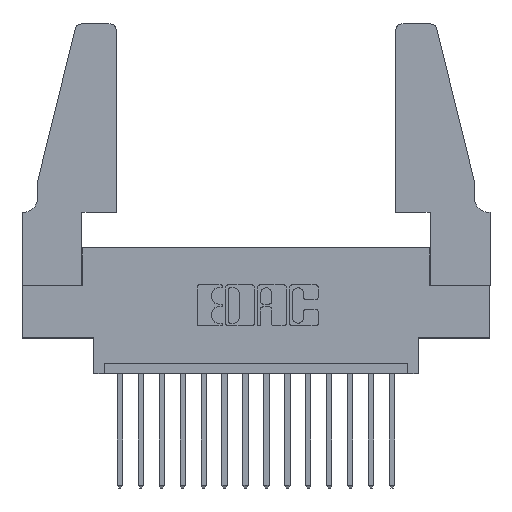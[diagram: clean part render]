
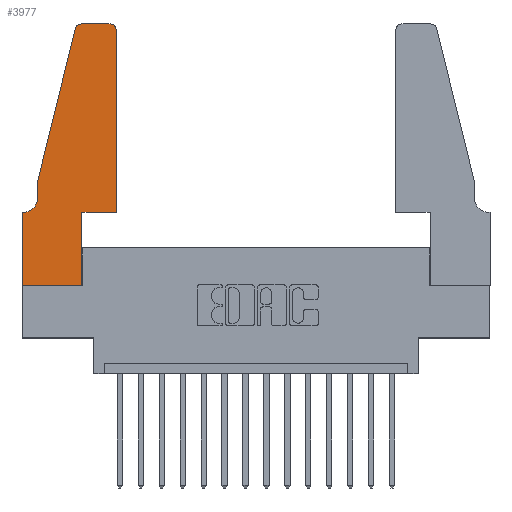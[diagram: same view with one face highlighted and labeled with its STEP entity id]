
A CAD part, top view. The second image highlights one B-rep face of the part: STEP entity #3977.
In plain terms, the highlighted planar face has unit normal (0, 0, 1).
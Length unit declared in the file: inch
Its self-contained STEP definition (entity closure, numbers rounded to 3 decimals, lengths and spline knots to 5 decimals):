
#444 = ORIENTED_EDGE ( 'NONE', *, *, #12407, .T. ) ;
#450 = CARTESIAN_POINT ( 'NONE',  ( 0.0755, 0.5, 0.37 ) ) ;
#571 = VERTEX_POINT ( 'NONE', #15454 ) ;
#788 = DIRECTION ( 'NONE',  ( -1., 0., 0. ) ) ;
#810 = VERTEX_POINT ( 'NONE', #12180 ) ;
#902 = CARTESIAN_POINT ( 'NONE',  ( 0.0755, 0.35, 0.37 ) ) ;
#979 = VERTEX_POINT ( 'NONE', #6836 ) ;
#1554 = CIRCLE ( 'NONE', #11083, 0.03 ) ;
#1864 = CARTESIAN_POINT ( 'NONE',  ( 0., 0., 0.37 ) ) ;
#2196 = LINE ( 'NONE', #10631, #14608 ) ;
#2213 = VECTOR ( 'NONE', #13676, 39.37008 ) ;
#2278 = CARTESIAN_POINT ( 'NONE',  ( 0.0055, 0.35, 0.37 ) ) ;
#2489 = DIRECTION ( 'NONE',  ( 0., 1., 0. ) ) ;
#3159 = CARTESIAN_POINT ( 'NONE',  ( 0.0755, 0.5, 0.37 ) ) ;
#3360 = EDGE_CURVE ( 'NONE', #9007, #979, #4590, .T. ) ;
#3392 = LINE ( 'NONE', #11049, #16000 ) ;
#3404 = EDGE_LOOP ( 'NONE', ( #8629, #16178, #14666, #444, #14325, #9494, #13981, #5302, #7642, #16197, #7687, #7142 ) ) ;
#3460 = CARTESIAN_POINT ( 'NONE',  ( 0.4505, 0.35, 0.37 ) ) ;
#3774 = AXIS2_PLACEMENT_3D ( 'NONE', #11562, #12553, #8917 ) ;
#3889 = CARTESIAN_POINT ( 'NONE',  ( 0.284, 1.25, 0.37 ) ) ;
#3894 = VERTEX_POINT ( 'NONE', #2278 ) ;
#3977 = ADVANCED_FACE ( 'NONE', ( #8327 ), #11458, .T. ) ;
#4134 = DIRECTION ( 'NONE',  ( 0., -1., 0. ) ) ;
#4146 = VECTOR ( 'NONE', #12476, 39.37008 ) ;
#4385 = CARTESIAN_POINT ( 'NONE',  ( 0.4205, 1.22, 0.37 ) ) ;
#4590 = CIRCLE ( 'NONE', #13576, 0.03 ) ;
#4602 = EDGE_CURVE ( 'NONE', #3894, #571, #8526, .T. ) ;
#4717 = CARTESIAN_POINT ( 'NONE',  ( 0.0755, 0.42, 0.37 ) ) ;
#4989 = CARTESIAN_POINT ( 'NONE',  ( 0.4505, 1.22, 0.37 ) ) ;
#5302 = ORIENTED_EDGE ( 'NONE', *, *, #15506, .T. ) ;
#5590 = LINE ( 'NONE', #1864, #2213 ) ;
#5667 = EDGE_CURVE ( 'NONE', #12551, #9007, #15120, .T. ) ;
#5698 = DIRECTION ( 'NONE',  ( 0., -1., 0. ) ) ;
#6191 = CIRCLE ( 'NONE', #9020, 0.07 ) ;
#6420 = VECTOR ( 'NONE', #11689, 39.37008 ) ;
#6467 = VECTOR ( 'NONE', #8378, 39.37008 ) ;
#6721 = VERTEX_POINT ( 'NONE', #4989 ) ;
#6766 = DIRECTION ( 'NONE',  ( 1., 0., 0. ) ) ;
#6836 = CARTESIAN_POINT ( 'NONE',  ( 0.25487, 1.22718, 0.37 ) ) ;
#7010 = VERTEX_POINT ( 'NONE', #12358 ) ;
#7142 = ORIENTED_EDGE ( 'NONE', *, *, #16295, .T. ) ;
#7149 = EDGE_CURVE ( 'NONE', #8238, #6721, #13042, .T. ) ;
#7272 = VECTOR ( 'NONE', #5698, 39.37008 ) ;
#7297 = DIRECTION ( 'NONE',  ( 1., 0., 0. ) ) ;
#7642 = ORIENTED_EDGE ( 'NONE', *, *, #7928, .T. ) ;
#7687 = ORIENTED_EDGE ( 'NONE', *, *, #7149, .T. ) ;
#7867 = LINE ( 'NONE', #3159, #6467 ) ;
#7928 = EDGE_CURVE ( 'NONE', #810, #9822, #14039, .T. ) ;
#8238 = VERTEX_POINT ( 'NONE', #3460 ) ;
#8327 = FACE_OUTER_BOUND ( 'NONE', #3404, .T. ) ;
#8378 = DIRECTION ( 'NONE',  ( -0.239, -0.971, 0. ) ) ;
#8393 = DIRECTION ( 'NONE',  ( 0., 0., -1. ) ) ;
#8526 = LINE ( 'NONE', #902, #4146 ) ;
#8551 = EDGE_CURVE ( 'NONE', #12487, #3894, #6191, .T. ) ;
#8629 = ORIENTED_EDGE ( 'NONE', *, *, #5667, .T. ) ;
#8897 = EDGE_CURVE ( 'NONE', #571, #12435, #2196, .T. ) ;
#8917 = DIRECTION ( 'NONE',  ( 1., 0., 0. ) ) ;
#9007 = VERTEX_POINT ( 'NONE', #3889 ) ;
#9020 = AXIS2_PLACEMENT_3D ( 'NONE', #15032, #8393, #12472 ) ;
#9494 = ORIENTED_EDGE ( 'NONE', *, *, #4602, .T. ) ;
#9822 = VERTEX_POINT ( 'NONE', #13778 ) ;
#10172 = CARTESIAN_POINT ( 'NONE',  ( 0.4505, 0.35, 0.37 ) ) ;
#10276 = EDGE_CURVE ( 'NONE', #9822, #8238, #3392, .T. ) ;
#10631 = CARTESIAN_POINT ( 'NONE',  ( 0., 0., 0.37 ) ) ;
#11049 = CARTESIAN_POINT ( 'NONE',  ( 0.4505, 0.35, 0.37 ) ) ;
#11083 = AXIS2_PLACEMENT_3D ( 'NONE', #4385, #13176, #6766 ) ;
#11458 = PLANE ( 'NONE',  #3774 ) ;
#11562 = CARTESIAN_POINT ( 'NONE',  ( 0., 0.35, 0.37 ) ) ;
#11689 = DIRECTION ( 'NONE',  ( 0., 1., 0. ) ) ;
#12035 = DIRECTION ( 'NONE',  ( 1., 0., 0. ) ) ;
#12180 = CARTESIAN_POINT ( 'NONE',  ( 0.2865, 0., 0.37 ) ) ;
#12242 = VECTOR ( 'NONE', #2489, 39.37008 ) ;
#12358 = CARTESIAN_POINT ( 'NONE',  ( 0.0755, 0.5, 0.37 ) ) ;
#12407 = EDGE_CURVE ( 'NONE', #7010, #12487, #15523, .T. ) ;
#12435 = VERTEX_POINT ( 'NONE', #15975 ) ;
#12470 = VECTOR ( 'NONE', #788, 39.37008 ) ;
#12472 = DIRECTION ( 'NONE',  ( -1., 0., 0. ) ) ;
#12476 = DIRECTION ( 'NONE',  ( -1., 0., 0. ) ) ;
#12487 = VERTEX_POINT ( 'NONE', #4717 ) ;
#12551 = VERTEX_POINT ( 'NONE', #15083 ) ;
#12553 = DIRECTION ( 'NONE',  ( 0., 0., 1. ) ) ;
#12904 = CARTESIAN_POINT ( 'NONE',  ( 0.2865, 0.35, 0.37 ) ) ;
#13042 = LINE ( 'NONE', #10172, #12242 ) ;
#13176 = DIRECTION ( 'NONE',  ( 0., 0., 1. ) ) ;
#13576 = AXIS2_PLACEMENT_3D ( 'NONE', #14892, #16112, #7297 ) ;
#13676 = DIRECTION ( 'NONE',  ( 1., 0., 0. ) ) ;
#13677 = EDGE_CURVE ( 'NONE', #979, #7010, #7867, .T. ) ;
#13778 = CARTESIAN_POINT ( 'NONE',  ( 0.2865, 0.35, 0.37 ) ) ;
#13981 = ORIENTED_EDGE ( 'NONE', *, *, #8897, .T. ) ;
#14039 = LINE ( 'NONE', #12904, #6420 ) ;
#14325 = ORIENTED_EDGE ( 'NONE', *, *, #8551, .T. ) ;
#14608 = VECTOR ( 'NONE', #4134, 39.37008 ) ;
#14666 = ORIENTED_EDGE ( 'NONE', *, *, #13677, .T. ) ;
#14892 = CARTESIAN_POINT ( 'NONE',  ( 0.284, 1.22, 0.37 ) ) ;
#15032 = CARTESIAN_POINT ( 'NONE',  ( 0.0055, 0.42, 0.37 ) ) ;
#15083 = CARTESIAN_POINT ( 'NONE',  ( 0.4205, 1.25, 0.37 ) ) ;
#15120 = LINE ( 'NONE', #15826, #12470 ) ;
#15454 = CARTESIAN_POINT ( 'NONE',  ( 0., 0.35, 0.37 ) ) ;
#15506 = EDGE_CURVE ( 'NONE', #12435, #810, #5590, .T. ) ;
#15523 = LINE ( 'NONE', #450, #7272 ) ;
#15826 = CARTESIAN_POINT ( 'NONE',  ( 0.2605, 1.25, 0.37 ) ) ;
#15975 = CARTESIAN_POINT ( 'NONE',  ( 0., 0., 0.37 ) ) ;
#16000 = VECTOR ( 'NONE', #12035, 39.37008 ) ;
#16112 = DIRECTION ( 'NONE',  ( 0., 0., 1. ) ) ;
#16178 = ORIENTED_EDGE ( 'NONE', *, *, #3360, .T. ) ;
#16197 = ORIENTED_EDGE ( 'NONE', *, *, #10276, .T. ) ;
#16295 = EDGE_CURVE ( 'NONE', #6721, #12551, #1554, .T. ) ;
